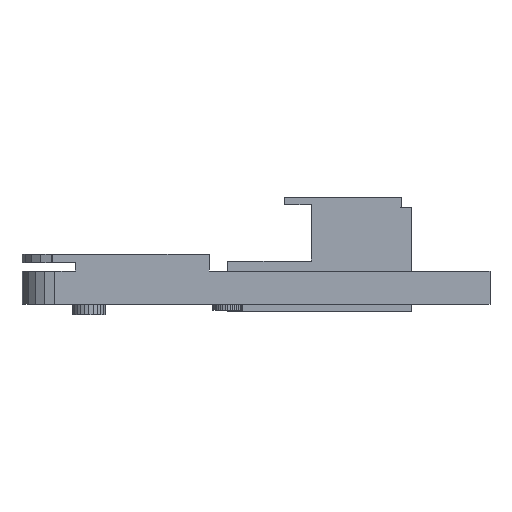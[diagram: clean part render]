
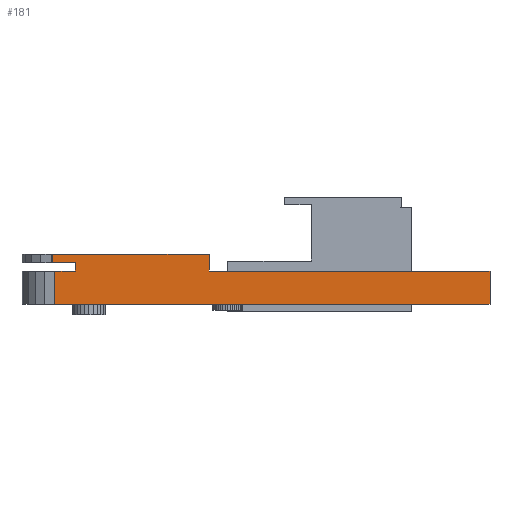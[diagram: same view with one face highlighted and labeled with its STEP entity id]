
A CAD part, front view. The second image highlights one B-rep face of the part: STEP entity #181.
In plain terms, the highlighted planar face has unit normal (0, -1, 0).
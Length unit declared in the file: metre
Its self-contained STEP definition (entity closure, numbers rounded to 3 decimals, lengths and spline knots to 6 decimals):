
#181=ADVANCED_FACE('0:987',(#666),#667,.T.);
#666=FACE_OUTER_BOUND('',#1443,.T.);
#667=PLANE('',#1444);
#1443=EDGE_LOOP('',(#2963,#2964,#2965,#2966,#2967,#2968,#2969,#2970,#2971,#2972));
#1444=AXIS2_PLACEMENT_3D('',#2973,#2974,#2975);
#2963=ORIENTED_EDGE('',*,*,#5568,.F.);
#2964=ORIENTED_EDGE('',*,*,#5698,.F.);
#2965=ORIENTED_EDGE('',*,*,#5645,.T.);
#2966=ORIENTED_EDGE('',*,*,#5699,.T.);
#2967=ORIENTED_EDGE('',*,*,#5552,.F.);
#2968=ORIENTED_EDGE('',*,*,#5696,.T.);
#2969=ORIENTED_EDGE('',*,*,#5700,.T.);
#2970=ORIENTED_EDGE('',*,*,#5701,.T.);
#2971=ORIENTED_EDGE('',*,*,#5702,.F.);
#2972=ORIENTED_EDGE('',*,*,#5691,.F.);
#2973=CARTESIAN_POINT('',(-0.036452,0.,0.015875));
#2974=DIRECTION('',(0.0,-1.,0.));
#2975=DIRECTION('',(0.0,0.,-1.));
#5552=EDGE_CURVE('0:1398',#6802,#6804,#6805,.T.);
#5568=EDGE_CURVE('0:1446',#6834,#6836,#6837,.T.);
#5645=EDGE_CURVE('0:1677',#6987,#6985,#6988,.T.);
#5691=EDGE_CURVE('0:1815',#6836,#7061,#7065,.T.);
#5696=EDGE_CURVE('0:1830',#6802,#7073,#7074,.T.);
#5698=EDGE_CURVE('0:1836',#6987,#6834,#7076,.T.);
#5699=EDGE_CURVE('0:1839',#6985,#6804,#7077,.T.);
#5700=EDGE_CURVE('0:1842',#7073,#7078,#7079,.T.);
#5701=EDGE_CURVE('0:1845',#7078,#7080,#7081,.T.);
#5702=EDGE_CURVE('0:1848',#7061,#7080,#7082,.T.);
#6802=VERTEX_POINT('',#8852);
#6804=VERTEX_POINT('',#8855);
#6805=LINE('',#8856,#8857);
#6834=VERTEX_POINT('',#8900);
#6836=VERTEX_POINT('',#8903);
#6837=LINE('',#8904,#8905);
#6985=VERTEX_POINT('',#9128);
#6987=VERTEX_POINT('',#9131);
#6988=LINE('',#9132,#9133);
#7061=VERTEX_POINT('',#9249);
#7065=LINE('',#9255,#9256);
#7073=VERTEX_POINT('',#9268);
#7074=LINE('',#9269,#9270);
#7076=LINE('',#9273,#9274);
#7077=LINE('',#9275,#9276);
#7078=VERTEX_POINT('',#9277);
#7079=LINE('',#9278,#9279);
#7080=VERTEX_POINT('',#9280);
#7081=LINE('',#9281,#9282);
#7082=LINE('',#9283,#9284);
#8852=CARTESIAN_POINT('',(0.014348,0.,0.015875));
#8855=CARTESIAN_POINT('',(0.121028,0.,0.015875));
#8856=CARTESIAN_POINT('',(0.014348,0.,0.015875));
#8857=VECTOR('',#11350,1.0);
#8900=CARTESIAN_POINT('',(-0.044326,0.,0.015875));
#8903=CARTESIAN_POINT('',(-0.036452,0.,0.015875));
#8904=CARTESIAN_POINT('',(-0.044326,0.,0.015875));
#8905=VECTOR('',#11366,1.0);
#9128=CARTESIAN_POINT('',(0.121028,0.,0.003175));
#9131=CARTESIAN_POINT('',(-0.044326,0.,0.003175));
#9132=CARTESIAN_POINT('',(-0.044326,0.,0.003175));
#9133=VECTOR('',#11443,1.0);
#9249=CARTESIAN_POINT('',(-0.036452,0.,0.01905));
#9255=CARTESIAN_POINT('',(-0.036452,0.,0.015875));
#9256=VECTOR('',#11489,1.0);
#9268=CARTESIAN_POINT('',(0.014348,0.,0.022225));
#9269=CARTESIAN_POINT('',(0.014348,0.,0.015875));
#9270=VECTOR('',#11494,1.0);
#9273=CARTESIAN_POINT('',(-0.044326,0.,0.003175));
#9274=VECTOR('',#11496,1.0);
#9275=CARTESIAN_POINT('',(0.121028,0.,0.003175));
#9276=VECTOR('',#11497,1.0);
#9277=CARTESIAN_POINT('',(-0.045206,0.,0.022225));
#9278=CARTESIAN_POINT('',(0.014348,0.,0.022225));
#9279=VECTOR('',#11498,1.0);
#9280=CARTESIAN_POINT('',(-0.045206,0.,0.01905));
#9281=CARTESIAN_POINT('',(-0.045206,0.,0.022225));
#9282=VECTOR('',#11499,1.0);
#9283=CARTESIAN_POINT('',(-0.036452,0.,0.01905));
#9284=VECTOR('',#11500,1.0);
#11350=DIRECTION('',(1.0,0.0,0.0));
#11366=DIRECTION('',(1.0,0.0,0.0));
#11443=DIRECTION('',(1.0,0.0,0.0));
#11489=DIRECTION('',(0.0,0.0,1.0));
#11494=DIRECTION('',(0.0,0.,1.));
#11496=DIRECTION('',(0.0,0.,1.));
#11497=DIRECTION('',(0.0,0.,1.));
#11498=DIRECTION('',(-1.0,0.0,0.0));
#11499=DIRECTION('',(0.0,0.,-1.));
#11500=DIRECTION('',(-1.0,0.0,0.0));
